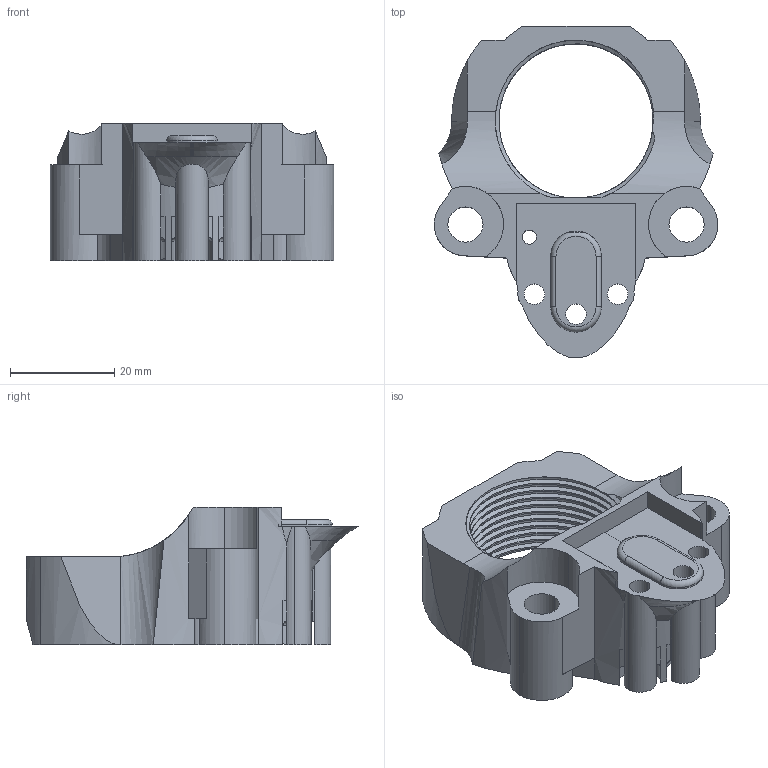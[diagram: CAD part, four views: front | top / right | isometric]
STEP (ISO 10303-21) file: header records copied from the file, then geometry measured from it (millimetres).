
FILE_DESCRIPTION (( 'STEP AP203' ), '1' );
FILE_NAME ('BufferTower.STEP', '2019-09-03T07:06:12', ( '' ), ( '' ), 'SwSTEP 2.0', 'SolidWorks 2018', '' );
FILE_SCHEMA (( 'CONFIG_CONTROL_DESIGN' ));
Length unit declared in the file: millimetre
Products named in the file (1): BufferTower
Bounding box: 54.43 x 63.72 x 26.43 mm (x, y, z)
Volume: 27354.8 mm3; surface area: 12793.1 mm2
Topology: 1 solids, 1 shells, 188 faces, 530 edges, 344 vertices
Faces by surface type: cylinder 93, plane 56, bspline 25, torus 8, cone 6
Entity records: 14243 total; most frequent: CARTESIAN_POINT 9602, ORIENTED_EDGE 1060, DIRECTION 848, EDGE_CURVE 530, VERTEX_POINT 344, AXIS2_PLACEMENT_3D 317, VECTOR 214, LINE 214
